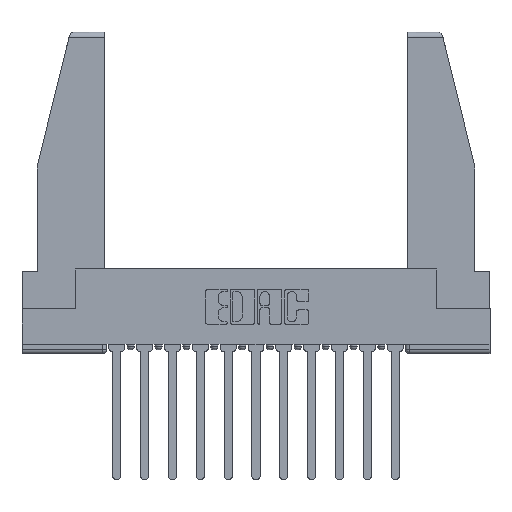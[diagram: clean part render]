
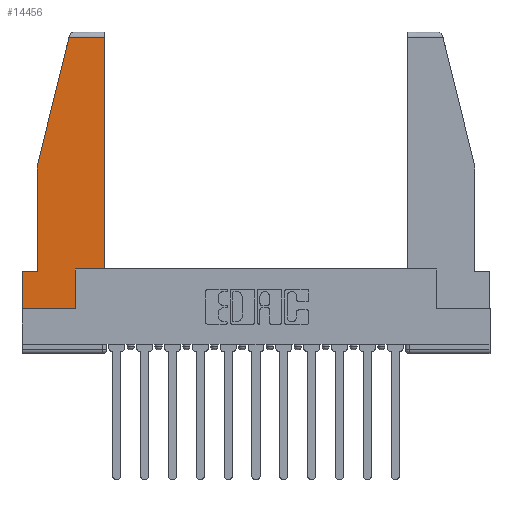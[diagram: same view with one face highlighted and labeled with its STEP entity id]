
A CAD part, top view. The second image highlights one B-rep face of the part: STEP entity #14456.
In plain terms, the highlighted planar face has unit normal (0, 0, 1).
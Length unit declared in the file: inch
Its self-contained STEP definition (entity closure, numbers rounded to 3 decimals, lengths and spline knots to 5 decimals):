
#73 = CARTESIAN_POINT ( 'NONE',  ( 0., 0.21, 0. ) ) ;
#235 = DIRECTION ( 'NONE',  ( 0., -1., 0. ) ) ;
#466 = CARTESIAN_POINT ( 'NONE',  ( 0.2636, 1.52, 0. ) ) ;
#488 = VERTEX_POINT ( 'NONE', #8180 ) ;
#500 = EDGE_LOOP ( 'NONE', ( #8215, #3723, #6886, #12273, #13401, #11435, #9642, #14039, #14663 ) ) ;
#833 = EDGE_CURVE ( 'NONE', #6769, #2382, #14045, .T. ) ;
#867 = VECTOR ( 'NONE', #1452, 39.37008 ) ;
#871 = VECTOR ( 'NONE', #235, 39.37008 ) ;
#897 = EDGE_CURVE ( 'NONE', #4894, #6769, #12050, .T. ) ;
#1452 = DIRECTION ( 'NONE',  ( -1., 0., 0. ) ) ;
#1567 = CARTESIAN_POINT ( 'NONE',  ( 0.271, 1.55, 0. ) ) ;
#1646 = DIRECTION ( 'NONE',  ( -0.239, -0.971, 0. ) ) ;
#1663 = DIRECTION ( 'NONE',  ( 1., 0., 0. ) ) ;
#1744 = FACE_OUTER_BOUND ( 'NONE', #500, .T. ) ;
#1759 = LINE ( 'NONE', #3271, #2139 ) ;
#1815 = DIRECTION ( 'NONE',  ( 0., 1., 0. ) ) ;
#1908 = DIRECTION ( 'NONE',  ( 1., 0., 0. ) ) ;
#2139 = VECTOR ( 'NONE', #8081, 39.37008 ) ;
#2382 = VERTEX_POINT ( 'NONE', #73 ) ;
#2403 = CARTESIAN_POINT ( 'NONE',  ( 0.461, 0.223, 0. ) ) ;
#2863 = CARTESIAN_POINT ( 'NONE',  ( 0., 0., 0. ) ) ;
#2918 = VECTOR ( 'NONE', #1815, 39.37008 ) ;
#2943 = CARTESIAN_POINT ( 'NONE',  ( 0., 0., 0. ) ) ;
#3076 = VERTEX_POINT ( 'NONE', #10495 ) ;
#3179 = CARTESIAN_POINT ( 'NONE',  ( 0., 0.21, 0. ) ) ;
#3271 = CARTESIAN_POINT ( 'NONE',  ( 0., 0., 0. ) ) ;
#3723 = ORIENTED_EDGE ( 'NONE', *, *, #5514, .T. ) ;
#4228 = CARTESIAN_POINT ( 'NONE',  ( 0.297, 0., 0. ) ) ;
#4853 = CARTESIAN_POINT ( 'NONE',  ( 0.086, 0.8, 0. ) ) ;
#4894 = VERTEX_POINT ( 'NONE', #4853 ) ;
#5354 = DIRECTION ( 'NONE',  ( -1., 0., 0. ) ) ;
#5474 = LINE ( 'NONE', #9172, #2918 ) ;
#5514 = EDGE_CURVE ( 'NONE', #15234, #8916, #12884, .T. ) ;
#6191 = LINE ( 'NONE', #7449, #871 ) ;
#6219 = VECTOR ( 'NONE', #1646, 39.37008 ) ;
#6523 = CARTESIAN_POINT ( 'NONE',  ( 0.297, 0.223, 0. ) ) ;
#6769 = VERTEX_POINT ( 'NONE', #15407 ) ;
#6830 = AXIS2_PLACEMENT_3D ( 'NONE', #2943, #7903, #1663 ) ;
#6886 = ORIENTED_EDGE ( 'NONE', *, *, #9603, .T. ) ;
#6896 = VERTEX_POINT ( 'NONE', #2403 ) ;
#7449 = CARTESIAN_POINT ( 'NONE',  ( 0., 0.21, 0. ) ) ;
#7609 = LINE ( 'NONE', #6523, #14096 ) ;
#7903 = DIRECTION ( 'NONE',  ( 0., 0., 1. ) ) ;
#8081 = DIRECTION ( 'NONE',  ( 1., 0., 0. ) ) ;
#8180 = CARTESIAN_POINT ( 'NONE',  ( 0.297, 0.223, 0. ) ) ;
#8215 = ORIENTED_EDGE ( 'NONE', *, *, #8967, .T. ) ;
#8657 = EDGE_CURVE ( 'NONE', #14406, #3076, #1759, .T. ) ;
#8804 = DIRECTION ( 'NONE',  ( 0., 1., 0. ) ) ;
#8843 = EDGE_CURVE ( 'NONE', #2382, #14406, #6191, .T. ) ;
#8916 = VERTEX_POINT ( 'NONE', #466 ) ;
#8949 = PLANE ( 'NONE',  #6830 ) ;
#8967 = EDGE_CURVE ( 'NONE', #6896, #15234, #5474, .T. ) ;
#9056 = CARTESIAN_POINT ( 'NONE',  ( 0., 1.52, 0. ) ) ;
#9172 = CARTESIAN_POINT ( 'NONE',  ( 0.461, 0.223, 0. ) ) ;
#9603 = EDGE_CURVE ( 'NONE', #8916, #4894, #12446, .T. ) ;
#9642 = ORIENTED_EDGE ( 'NONE', *, *, #8657, .T. ) ;
#10216 = VECTOR ( 'NONE', #5354, 39.37008 ) ;
#10493 = EDGE_CURVE ( 'NONE', #3076, #488, #12387, .T. ) ;
#10495 = CARTESIAN_POINT ( 'NONE',  ( 0.297, 0., 0. ) ) ;
#10616 = EDGE_CURVE ( 'NONE', #488, #6896, #7609, .T. ) ;
#10761 = DIRECTION ( 'NONE',  ( 0., -1., 0. ) ) ;
#10766 = VECTOR ( 'NONE', #10761, 39.37008 ) ;
#10782 = VECTOR ( 'NONE', #8804, 39.37008 ) ;
#11435 = ORIENTED_EDGE ( 'NONE', *, *, #8843, .T. ) ;
#12050 = LINE ( 'NONE', #15530, #10766 ) ;
#12273 = ORIENTED_EDGE ( 'NONE', *, *, #897, .T. ) ;
#12387 = LINE ( 'NONE', #4228, #10782 ) ;
#12446 = LINE ( 'NONE', #1567, #6219 ) ;
#12884 = LINE ( 'NONE', #9056, #10216 ) ;
#13401 = ORIENTED_EDGE ( 'NONE', *, *, #833, .T. ) ;
#14039 = ORIENTED_EDGE ( 'NONE', *, *, #10493, .T. ) ;
#14045 = LINE ( 'NONE', #3179, #867 ) ;
#14096 = VECTOR ( 'NONE', #1908, 39.37008 ) ;
#14406 = VERTEX_POINT ( 'NONE', #2863 ) ;
#14456 = ADVANCED_FACE ( 'NONE', ( #1744 ), #8949, .T. ) ;
#14663 = ORIENTED_EDGE ( 'NONE', *, *, #10616, .T. ) ;
#14961 = CARTESIAN_POINT ( 'NONE',  ( 0.461, 1.52, 0. ) ) ;
#15234 = VERTEX_POINT ( 'NONE', #14961 ) ;
#15407 = CARTESIAN_POINT ( 'NONE',  ( 0.086, 0.21, 0. ) ) ;
#15530 = CARTESIAN_POINT ( 'NONE',  ( 0.086, 0.8, 0. ) ) ;
